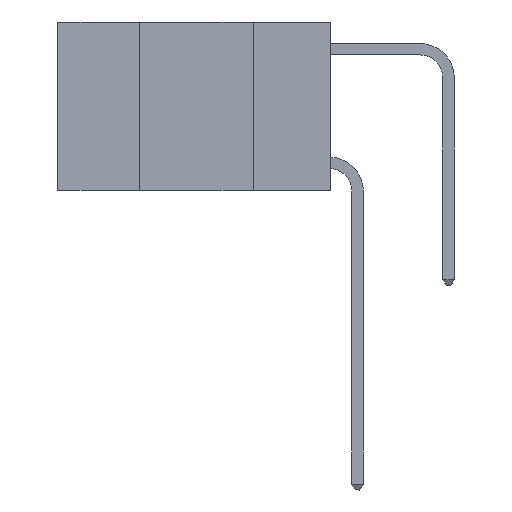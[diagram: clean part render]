
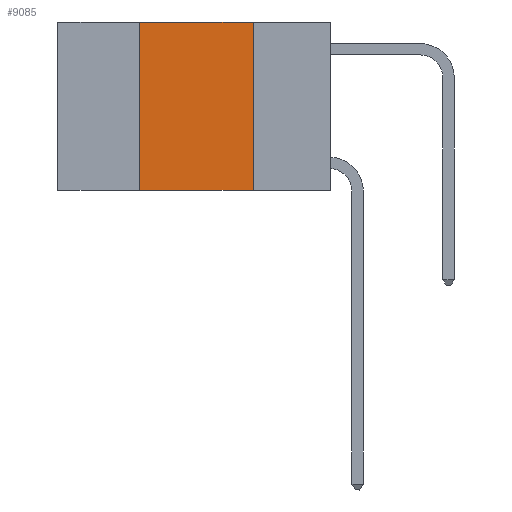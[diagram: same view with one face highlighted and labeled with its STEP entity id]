
A CAD part, left-side view. The second image highlights one B-rep face of the part: STEP entity #9085.
In plain terms, the highlighted planar face has unit normal (-1, 0, 0).
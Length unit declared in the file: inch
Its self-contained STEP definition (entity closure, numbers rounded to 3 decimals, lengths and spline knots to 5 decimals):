
#271 = CARTESIAN_POINT ( 'NONE',  ( 0., 0.42, 0. ) ) ;
#830 = CARTESIAN_POINT ( 'NONE',  ( 0., 0.42, 0. ) ) ;
#4662 = ORIENTED_EDGE ( 'NONE', *, *, #11804, .F. ) ;
#5585 = CARTESIAN_POINT ( 'NONE',  ( 0., 0.17, 0. ) ) ;
#5649 = EDGE_CURVE ( 'NONE', #19441, #13038, #8382, .T. ) ;
#5754 = DIRECTION ( 'NONE',  ( 0., 0., -1. ) ) ;
#6037 = ORIENTED_EDGE ( 'NONE', *, *, #14481, .F. ) ;
#6993 = EDGE_LOOP ( 'NONE', ( #25909, #4662, #6037, #17568 ) ) ;
#7532 = VERTEX_POINT ( 'NONE', #830 ) ;
#8382 = LINE ( 'NONE', #20181, #19857 ) ;
#9085 = ADVANCED_FACE ( 'NONE', ( #22319 ), #17265, .F. ) ;
#9613 = DIRECTION ( 'NONE',  ( 0., 0., 1. ) ) ;
#10329 = VERTEX_POINT ( 'NONE', #5585 ) ;
#11804 = EDGE_CURVE ( 'NONE', #7532, #10329, #28825, .T. ) ;
#12871 = VECTOR ( 'NONE', #13346, 39.37008 ) ;
#13038 = VERTEX_POINT ( 'NONE', #28056 ) ;
#13043 = CARTESIAN_POINT ( 'NONE',  ( 0., 0.17, 0. ) ) ;
#13346 = DIRECTION ( 'NONE',  ( 0., 0., -1. ) ) ;
#14201 = AXIS2_PLACEMENT_3D ( 'NONE', #26796, #24175, #5754 ) ;
#14481 = EDGE_CURVE ( 'NONE', #19441, #7532, #21272, .T. ) ;
#17265 = PLANE ( 'NONE',  #14201 ) ;
#17568 = ORIENTED_EDGE ( 'NONE', *, *, #5649, .T. ) ;
#18961 = CARTESIAN_POINT ( 'NONE',  ( 0., 0.42, -0.37 ) ) ;
#19441 = VERTEX_POINT ( 'NONE', #18961 ) ;
#19857 = VECTOR ( 'NONE', #24808, 39.37008 ) ;
#20181 = CARTESIAN_POINT ( 'NONE',  ( 0., 0.6, -0.37 ) ) ;
#21272 = LINE ( 'NONE', #271, #24410 ) ;
#21589 = CARTESIAN_POINT ( 'NONE',  ( 0., 0.6, 0. ) ) ;
#21842 = EDGE_CURVE ( 'NONE', #10329, #13038, #27173, .T. ) ;
#21887 = DIRECTION ( 'NONE',  ( 0., -1., 0. ) ) ;
#22319 = FACE_OUTER_BOUND ( 'NONE', #6993, .T. ) ;
#24175 = DIRECTION ( 'NONE',  ( 1., 0., 0. ) ) ;
#24410 = VECTOR ( 'NONE', #9613, 39.37008 ) ;
#24808 = DIRECTION ( 'NONE',  ( 0., -1., 0. ) ) ;
#25909 = ORIENTED_EDGE ( 'NONE', *, *, #21842, .F. ) ;
#26546 = VECTOR ( 'NONE', #21887, 39.37008 ) ;
#26796 = CARTESIAN_POINT ( 'NONE',  ( 0., 0.6, 0. ) ) ;
#27173 = LINE ( 'NONE', #13043, #12871 ) ;
#28056 = CARTESIAN_POINT ( 'NONE',  ( 0., 0.17, -0.37 ) ) ;
#28825 = LINE ( 'NONE', #21589, #26546 ) ;
